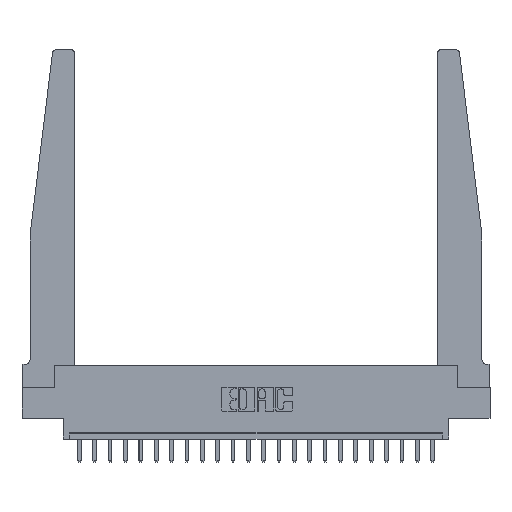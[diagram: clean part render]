
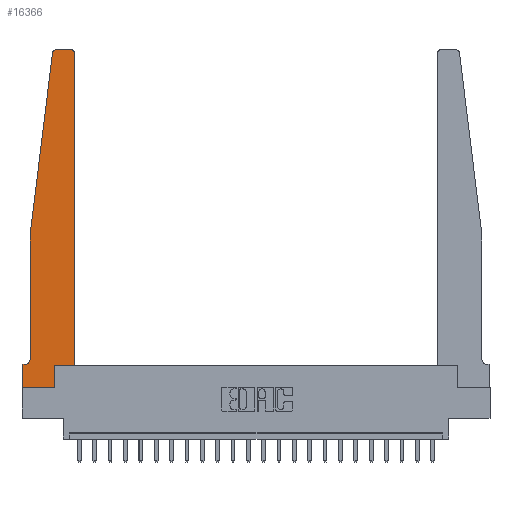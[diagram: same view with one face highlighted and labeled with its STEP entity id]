
A CAD part, top view. The second image highlights one B-rep face of the part: STEP entity #16366.
In plain terms, the highlighted planar face has unit normal (0, 0, 1).
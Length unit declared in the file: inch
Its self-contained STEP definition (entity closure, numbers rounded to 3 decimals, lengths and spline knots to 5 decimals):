
#278 = DIRECTION ( 'NONE',  ( 0., 1., 0. ) ) ;
#341 = PLANE ( 'NONE',  #14889 ) ;
#896 = EDGE_CURVE ( 'NONE', #3858, #7909, #7432, .T. ) ;
#1015 = CARTESIAN_POINT ( 'NONE',  ( 0.27653, 2.75, 0.37 ) ) ;
#1529 = EDGE_CURVE ( 'NONE', #14591, #21144, #5846, .T. ) ;
#1688 = CARTESIAN_POINT ( 'NONE',  ( 0.2605, 0.18, 0.37 ) ) ;
#1760 = CARTESIAN_POINT ( 'NONE',  ( 0.27653, 2.72, 0.37 ) ) ;
#1880 = DIRECTION ( 'NONE',  ( 0., 0., 1. ) ) ;
#2052 = ORIENTED_EDGE ( 'NONE', *, *, #18881, .T. ) ;
#2240 = LINE ( 'NONE', #11123, #22381 ) ;
#2452 = VECTOR ( 'NONE', #19897, 39.37008 ) ;
#2618 = VERTEX_POINT ( 'NONE', #9042 ) ;
#2716 = ORIENTED_EDGE ( 'NONE', *, *, #3125, .T. ) ;
#2805 = CARTESIAN_POINT ( 'NONE',  ( 0.395, 2.75, 0.37 ) ) ;
#2966 = VERTEX_POINT ( 'NONE', #12026 ) ;
#3113 = CARTESIAN_POINT ( 'NONE',  ( 0.425, 0.18, 0.37 ) ) ;
#3125 = EDGE_CURVE ( 'NONE', #21144, #2966, #16149, .T. ) ;
#3478 = VECTOR ( 'NONE', #9182, 39.37008 ) ;
#3842 = DIRECTION ( 'NONE',  ( 0., -1., 0. ) ) ;
#3858 = VERTEX_POINT ( 'NONE', #21366 ) ;
#4486 = DIRECTION ( 'NONE',  ( 0., 0., -1. ) ) ;
#4555 = VERTEX_POINT ( 'NONE', #19006 ) ;
#5049 = CARTESIAN_POINT ( 'NONE',  ( 0.065, 1.25, 0.37 ) ) ;
#5583 = ORIENTED_EDGE ( 'NONE', *, *, #21384, .T. ) ;
#5846 = LINE ( 'NONE', #19411, #3478 ) ;
#6216 = VECTOR ( 'NONE', #3842, 39.37008 ) ;
#6331 = EDGE_CURVE ( 'NONE', #8768, #14591, #9629, .T. ) ;
#6376 = ORIENTED_EDGE ( 'NONE', *, *, #13487, .T. ) ;
#7344 = CARTESIAN_POINT ( 'NONE',  ( 0., 0., 0.37 ) ) ;
#7432 = CIRCLE ( 'NONE', #10375, 0.03 ) ;
#7648 = DIRECTION ( 'NONE',  ( 1., 0., 0. ) ) ;
#7717 = DIRECTION ( 'NONE',  ( 0., 0., 1. ) ) ;
#7909 = VERTEX_POINT ( 'NONE', #2805 ) ;
#7928 = ORIENTED_EDGE ( 'NONE', *, *, #6331, .T. ) ;
#7944 = DIRECTION ( 'NONE',  ( 1., 0., 0. ) ) ;
#8202 = CARTESIAN_POINT ( 'NONE',  ( 0.25, 2.75, 0.37 ) ) ;
#8228 = CARTESIAN_POINT ( 'NONE',  ( 0.24675, 2.72367, 0.37 ) ) ;
#8768 = VERTEX_POINT ( 'NONE', #1015 ) ;
#9042 = CARTESIAN_POINT ( 'NONE',  ( 0., 0.1875, 0.37 ) ) ;
#9182 = DIRECTION ( 'NONE',  ( -0.122, -0.992, 0. ) ) ;
#9629 = CIRCLE ( 'NONE', #10366, 0.03 ) ;
#9675 = CARTESIAN_POINT ( 'NONE',  ( 0.425, 0.18, 0.37 ) ) ;
#10031 = EDGE_CURVE ( 'NONE', #2966, #14905, #11804, .T. ) ;
#10366 = AXIS2_PLACEMENT_3D ( 'NONE', #1760, #1880, #17773 ) ;
#10375 = AXIS2_PLACEMENT_3D ( 'NONE', #12967, #16643, #7648 ) ;
#11123 = CARTESIAN_POINT ( 'NONE',  ( 0.2605, 0.18, 0.37 ) ) ;
#11141 = DIRECTION ( 'NONE',  ( 0., 1., 0. ) ) ;
#11177 = DIRECTION ( 'NONE',  ( 1., 0., 0. ) ) ;
#11261 = CARTESIAN_POINT ( 'NONE',  ( 0., 0., 0.37 ) ) ;
#11392 = EDGE_CURVE ( 'NONE', #22287, #3858, #16543, .T. ) ;
#11399 = CARTESIAN_POINT ( 'NONE',  ( 0.065, 0.1875, 0.37 ) ) ;
#11424 = VECTOR ( 'NONE', #21970, 39.37008 ) ;
#11545 = CARTESIAN_POINT ( 'NONE',  ( 0.015, 0.1875, 0.37 ) ) ;
#11773 = DIRECTION ( 'NONE',  ( -1., 0., 0. ) ) ;
#11804 = CIRCLE ( 'NONE', #12156, 0.05 ) ;
#11969 = DIRECTION ( 'NONE',  ( -1., 0., 0. ) ) ;
#12026 = CARTESIAN_POINT ( 'NONE',  ( 0.065, 0.2375, 0.37 ) ) ;
#12156 = AXIS2_PLACEMENT_3D ( 'NONE', #15193, #4486, #11969 ) ;
#12307 = EDGE_LOOP ( 'NONE', ( #19375, #7928, #17243, #2716, #20799, #6376, #19790, #5583, #2052, #12710, #20417, #18482 ) ) ;
#12519 = VECTOR ( 'NONE', #11141, 39.37008 ) ;
#12710 = ORIENTED_EDGE ( 'NONE', *, *, #15349, .T. ) ;
#12967 = CARTESIAN_POINT ( 'NONE',  ( 0.395, 2.72, 0.37 ) ) ;
#13007 = VECTOR ( 'NONE', #11773, 39.37008 ) ;
#13242 = DIRECTION ( 'NONE',  ( -1., 0., 0. ) ) ;
#13487 = EDGE_CURVE ( 'NONE', #14905, #2618, #19487, .T. ) ;
#13681 = VECTOR ( 'NONE', #13242, 39.37008 ) ;
#13684 = VERTEX_POINT ( 'NONE', #1688 ) ;
#14097 = VECTOR ( 'NONE', #7944, 39.37008 ) ;
#14591 = VERTEX_POINT ( 'NONE', #8228 ) ;
#14889 = AXIS2_PLACEMENT_3D ( 'NONE', #17949, #7717, #11177 ) ;
#14905 = VERTEX_POINT ( 'NONE', #11545 ) ;
#14919 = EDGE_CURVE ( 'NONE', #7909, #8768, #14996, .T. ) ;
#14996 = LINE ( 'NONE', #8202, #13007 ) ;
#15193 = CARTESIAN_POINT ( 'NONE',  ( 0.015, 0.2375, 0.37 ) ) ;
#15349 = EDGE_CURVE ( 'NONE', #13684, #22287, #21988, .T. ) ;
#16149 = LINE ( 'NONE', #17757, #6216 ) ;
#16366 = ADVANCED_FACE ( 'NONE', ( #19809 ), #341, .T. ) ;
#16543 = LINE ( 'NONE', #21615, #12519 ) ;
#16643 = DIRECTION ( 'NONE',  ( 0., 0., 1. ) ) ;
#17243 = ORIENTED_EDGE ( 'NONE', *, *, #1529, .T. ) ;
#17709 = VERTEX_POINT ( 'NONE', #21048 ) ;
#17757 = CARTESIAN_POINT ( 'NONE',  ( 0.065, 1.25, 0.37 ) ) ;
#17773 = DIRECTION ( 'NONE',  ( 1., 0., 0. ) ) ;
#17923 = LINE ( 'NONE', #7344, #2452 ) ;
#17949 = CARTESIAN_POINT ( 'NONE',  ( 0., 0.1875, 0.37 ) ) ;
#17959 = EDGE_CURVE ( 'NONE', #2618, #4555, #17923, .T. ) ;
#18162 = LINE ( 'NONE', #11261, #11424 ) ;
#18482 = ORIENTED_EDGE ( 'NONE', *, *, #896, .T. ) ;
#18881 = EDGE_CURVE ( 'NONE', #17709, #13684, #2240, .T. ) ;
#19006 = CARTESIAN_POINT ( 'NONE',  ( 0., 0., 0.37 ) ) ;
#19375 = ORIENTED_EDGE ( 'NONE', *, *, #14919, .T. ) ;
#19411 = CARTESIAN_POINT ( 'NONE',  ( 0.065, 1.25, 0.37 ) ) ;
#19487 = LINE ( 'NONE', #11399, #13681 ) ;
#19790 = ORIENTED_EDGE ( 'NONE', *, *, #17959, .T. ) ;
#19809 = FACE_OUTER_BOUND ( 'NONE', #12307, .T. ) ;
#19897 = DIRECTION ( 'NONE',  ( 0., -1., 0. ) ) ;
#20417 = ORIENTED_EDGE ( 'NONE', *, *, #11392, .T. ) ;
#20799 = ORIENTED_EDGE ( 'NONE', *, *, #10031, .T. ) ;
#21048 = CARTESIAN_POINT ( 'NONE',  ( 0.2605, 0., 0.37 ) ) ;
#21144 = VERTEX_POINT ( 'NONE', #5049 ) ;
#21366 = CARTESIAN_POINT ( 'NONE',  ( 0.425, 2.72, 0.37 ) ) ;
#21384 = EDGE_CURVE ( 'NONE', #4555, #17709, #18162, .T. ) ;
#21615 = CARTESIAN_POINT ( 'NONE',  ( 0.425, 0.18, 0.37 ) ) ;
#21970 = DIRECTION ( 'NONE',  ( 1., 0., 0. ) ) ;
#21988 = LINE ( 'NONE', #9675, #14097 ) ;
#22287 = VERTEX_POINT ( 'NONE', #3113 ) ;
#22381 = VECTOR ( 'NONE', #278, 39.37008 ) ;
